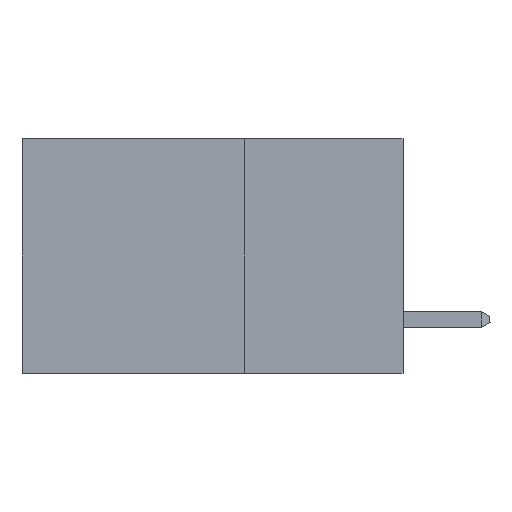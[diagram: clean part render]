
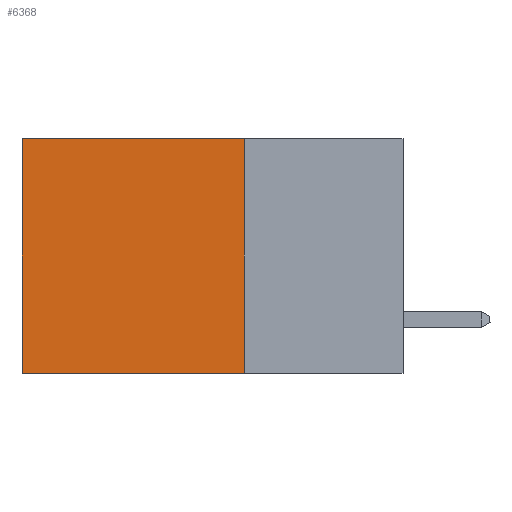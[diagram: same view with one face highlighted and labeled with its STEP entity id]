
A CAD part, left-side view. The second image highlights one B-rep face of the part: STEP entity #6368.
In plain terms, the highlighted planar face has unit normal (-1, 0, 0).
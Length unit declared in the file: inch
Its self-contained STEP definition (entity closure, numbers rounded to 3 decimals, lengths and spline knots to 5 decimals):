
#33 = EDGE_CURVE ( 'NONE', #3284, #2000, #5360, .T. ) ;
#37 = LINE ( 'NONE', #346, #1462 ) ;
#53 = VERTEX_POINT ( 'NONE', #11609 ) ;
#346 = CARTESIAN_POINT ( 'NONE',  ( 0.2875, 0.6, 0. ) ) ;
#505 = DIRECTION ( 'NONE',  ( 1., 0., 0. ) ) ;
#935 = CARTESIAN_POINT ( 'NONE',  ( 0.2875, 0.25, 0. ) ) ;
#1256 = CARTESIAN_POINT ( 'NONE',  ( 0.2875, 0.25, -0.37 ) ) ;
#1327 = DIRECTION ( 'NONE',  ( 0., 1., 0. ) ) ;
#1462 = VECTOR ( 'NONE', #13677, 39.37008 ) ;
#1618 = VERTEX_POINT ( 'NONE', #13645 ) ;
#2000 = VERTEX_POINT ( 'NONE', #4327 ) ;
#2550 = EDGE_LOOP ( 'NONE', ( #13933, #12721, #11840, #8731 ) ) ;
#2800 = EDGE_CURVE ( 'NONE', #2000, #53, #14119, .T. ) ;
#3284 = VERTEX_POINT ( 'NONE', #10749 ) ;
#4327 = CARTESIAN_POINT ( 'NONE',  ( 0.2875, 0.25, -0.37 ) ) ;
#4667 = EDGE_CURVE ( 'NONE', #1618, #53, #37, .T. ) ;
#5360 = LINE ( 'NONE', #13288, #12299 ) ;
#6122 = LINE ( 'NONE', #935, #9918 ) ;
#6368 = ADVANCED_FACE ( 'NONE', ( #12102 ), #13754, .F. ) ;
#8731 = ORIENTED_EDGE ( 'NONE', *, *, #8902, .T. ) ;
#8902 = EDGE_CURVE ( 'NONE', #3284, #1618, #6122, .T. ) ;
#9918 = VECTOR ( 'NONE', #1327, 39.37008 ) ;
#10381 = DIRECTION ( 'NONE',  ( 0., 0., -1. ) ) ;
#10434 = DIRECTION ( 'NONE',  ( 0., 0., -1. ) ) ;
#10478 = CARTESIAN_POINT ( 'NONE',  ( 0.2875, 0.25, 0. ) ) ;
#10749 = CARTESIAN_POINT ( 'NONE',  ( 0.2875, 0.25, 0. ) ) ;
#11187 = VECTOR ( 'NONE', #12311, 39.37008 ) ;
#11609 = CARTESIAN_POINT ( 'NONE',  ( 0.2875, 0.6, -0.37 ) ) ;
#11840 = ORIENTED_EDGE ( 'NONE', *, *, #33, .F. ) ;
#12102 = FACE_OUTER_BOUND ( 'NONE', #2550, .T. ) ;
#12299 = VECTOR ( 'NONE', #10381, 39.37008 ) ;
#12311 = DIRECTION ( 'NONE',  ( 0., 1., 0. ) ) ;
#12721 = ORIENTED_EDGE ( 'NONE', *, *, #2800, .F. ) ;
#13288 = CARTESIAN_POINT ( 'NONE',  ( 0.2875, 0.25, 0. ) ) ;
#13454 = AXIS2_PLACEMENT_3D ( 'NONE', #10478, #505, #10434 ) ;
#13645 = CARTESIAN_POINT ( 'NONE',  ( 0.2875, 0.6, 0. ) ) ;
#13677 = DIRECTION ( 'NONE',  ( 0., 0., -1. ) ) ;
#13754 = PLANE ( 'NONE',  #13454 ) ;
#13933 = ORIENTED_EDGE ( 'NONE', *, *, #4667, .T. ) ;
#14119 = LINE ( 'NONE', #1256, #11187 ) ;
